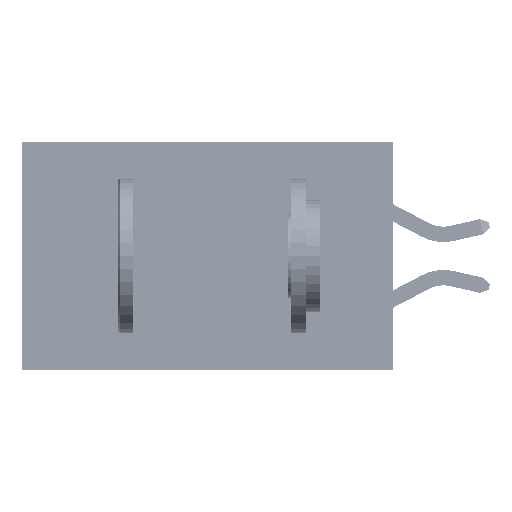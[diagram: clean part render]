
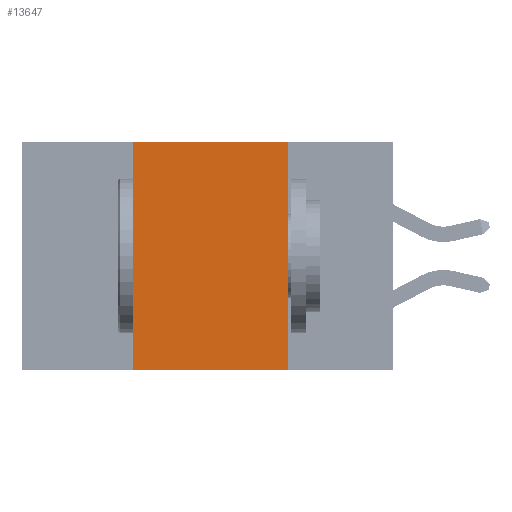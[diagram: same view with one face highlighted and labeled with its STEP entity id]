
A CAD part, left-side view. The second image highlights one B-rep face of the part: STEP entity #13647.
In plain terms, the highlighted planar face has unit normal (-1, 0, 0).
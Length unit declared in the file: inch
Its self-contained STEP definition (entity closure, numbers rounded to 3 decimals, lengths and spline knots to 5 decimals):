
#2375 = DIRECTION ( 'NONE',  ( 0., -1., 0. ) ) ;
#5408 = CARTESIAN_POINT ( 'NONE',  ( 0., 0.6, 0. ) ) ;
#8700 = EDGE_CURVE ( 'NONE', #37128, #19803, #44570, .T. ) ;
#10208 = CARTESIAN_POINT ( 'NONE',  ( 0., 0.42, -0.37 ) ) ;
#10526 = CARTESIAN_POINT ( 'NONE',  ( 0., 0.6, -0.37 ) ) ;
#10539 = CARTESIAN_POINT ( 'NONE',  ( 0., 0.17, -0.37 ) ) ;
#10620 = CARTESIAN_POINT ( 'NONE',  ( 0., 0.42, 0. ) ) ;
#10860 = DIRECTION ( 'NONE',  ( 0., -1., 0. ) ) ;
#12704 = ORIENTED_EDGE ( 'NONE', *, *, #20952, .F. ) ;
#13022 = CARTESIAN_POINT ( 'NONE',  ( 0., 0.42, 0. ) ) ;
#13102 = DIRECTION ( 'NONE',  ( 1., 0., 0. ) ) ;
#13169 = EDGE_CURVE ( 'NONE', #44733, #32629, #47998, .T. ) ;
#13647 = ADVANCED_FACE ( 'NONE', ( #21086 ), #49845, .F. ) ;
#15315 = AXIS2_PLACEMENT_3D ( 'NONE', #5408, #13102, #17532 ) ;
#16090 = LINE ( 'NONE', #10620, #36525 ) ;
#17532 = DIRECTION ( 'NONE',  ( 0., 0., -1. ) ) ;
#19803 = VERTEX_POINT ( 'NONE', #10539 ) ;
#20952 = EDGE_CURVE ( 'NONE', #32629, #19803, #39293, .T. ) ;
#21086 = FACE_OUTER_BOUND ( 'NONE', #30273, .T. ) ;
#21298 = CARTESIAN_POINT ( 'NONE',  ( 0., 0.17, 0. ) ) ;
#22898 = VECTOR ( 'NONE', #10860, 39.37008 ) ;
#23537 = ORIENTED_EDGE ( 'NONE', *, *, #8700, .T. ) ;
#26553 = ORIENTED_EDGE ( 'NONE', *, *, #13169, .F. ) ;
#26593 = EDGE_CURVE ( 'NONE', #37128, #44733, #16090, .T. ) ;
#29710 = VECTOR ( 'NONE', #50382, 39.37008 ) ;
#30273 = EDGE_LOOP ( 'NONE', ( #12704, #26553, #45821, #23537 ) ) ;
#30728 = VECTOR ( 'NONE', #2375, 39.37008 ) ;
#31082 = DIRECTION ( 'NONE',  ( 0., 0., 1. ) ) ;
#32629 = VERTEX_POINT ( 'NONE', #32931 ) ;
#32931 = CARTESIAN_POINT ( 'NONE',  ( 0., 0.17, 0. ) ) ;
#36525 = VECTOR ( 'NONE', #31082, 39.37008 ) ;
#37128 = VERTEX_POINT ( 'NONE', #10208 ) ;
#39293 = LINE ( 'NONE', #21298, #29710 ) ;
#43090 = CARTESIAN_POINT ( 'NONE',  ( 0., 0.6, 0. ) ) ;
#44570 = LINE ( 'NONE', #10526, #22898 ) ;
#44733 = VERTEX_POINT ( 'NONE', #13022 ) ;
#45821 = ORIENTED_EDGE ( 'NONE', *, *, #26593, .F. ) ;
#47998 = LINE ( 'NONE', #43090, #30728 ) ;
#49845 = PLANE ( 'NONE',  #15315 ) ;
#50382 = DIRECTION ( 'NONE',  ( 0., 0., -1. ) ) ;
